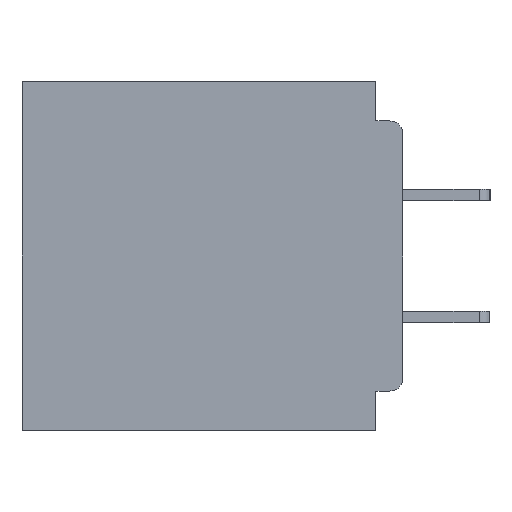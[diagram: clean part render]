
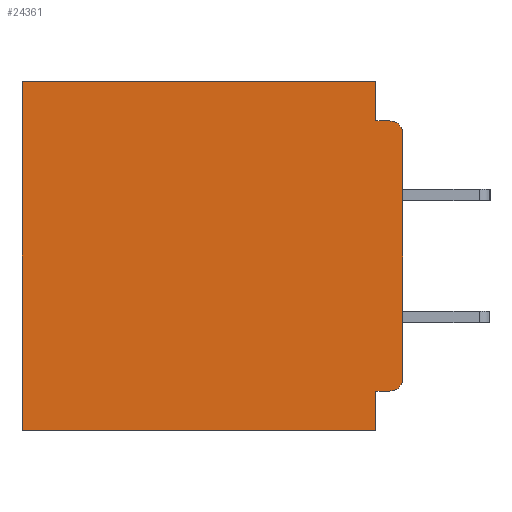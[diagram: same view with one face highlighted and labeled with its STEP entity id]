
A CAD part, left-side view. The second image highlights one B-rep face of the part: STEP entity #24361.
In plain terms, the highlighted planar face has unit normal (-1, 0, 0).
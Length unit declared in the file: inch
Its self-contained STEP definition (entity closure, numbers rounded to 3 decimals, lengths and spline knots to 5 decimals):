
#434 = EDGE_CURVE ( 'NONE', #15680, #1506, #31696, .T. ) ;
#1429 = CARTESIAN_POINT ( 'NONE',  ( 0.3, 0., -0.4 ) ) ;
#1449 = EDGE_CURVE ( 'NONE', #29071, #23700, #7052, .T. ) ;
#1506 = VERTEX_POINT ( 'NONE', #19476 ) ;
#1617 = DIRECTION ( 'NONE',  ( -1., 0., 0. ) ) ;
#1661 = CARTESIAN_POINT ( 'NONE',  ( 0.3, 0., -0.4 ) ) ;
#1756 = DIRECTION ( 'NONE',  ( 0., 0., -1. ) ) ;
#2538 = EDGE_LOOP ( 'NONE', ( #7887, #25222, #10624, #26122, #35601, #5634, #32492, #4267, #19746, #13804 ) ) ;
#2612 = CARTESIAN_POINT ( 'NONE',  ( 0.3, 0.031, -0.4 ) ) ;
#3013 = DIRECTION ( 'NONE',  ( -1., 0., 0. ) ) ;
#3930 = LINE ( 'NONE', #22100, #33946 ) ;
#4070 = EDGE_CURVE ( 'NONE', #23886, #24846, #15529, .T. ) ;
#4168 = EDGE_CURVE ( 'NONE', #24846, #30681, #34199, .T. ) ;
#4225 = CARTESIAN_POINT ( 'NONE',  ( 0.3, 0., -0.355 ) ) ;
#4267 = ORIENTED_EDGE ( 'NONE', *, *, #4168, .F. ) ;
#5488 = CARTESIAN_POINT ( 'NONE',  ( 0.3, 0., -0.045 ) ) ;
#5634 = ORIENTED_EDGE ( 'NONE', *, *, #24002, .T. ) ;
#5929 = DIRECTION ( 'NONE',  ( 0., 0., -1. ) ) ;
#6132 = LINE ( 'NONE', #1661, #36965 ) ;
#7052 = LINE ( 'NONE', #22260, #22573 ) ;
#7841 = VECTOR ( 'NONE', #13081, 39.37008 ) ;
#7887 = ORIENTED_EDGE ( 'NONE', *, *, #434, .F. ) ;
#8586 = AXIS2_PLACEMENT_3D ( 'NONE', #19026, #1617, #21970 ) ;
#8713 = DIRECTION ( 'NONE',  ( 0., 0., -1. ) ) ;
#9710 = VECTOR ( 'NONE', #11336, 39.37008 ) ;
#9947 = AXIS2_PLACEMENT_3D ( 'NONE', #20431, #3013, #23406 ) ;
#10624 = ORIENTED_EDGE ( 'NONE', *, *, #18194, .F. ) ;
#10672 = DIRECTION ( 'NONE',  ( 0., 0., -1. ) ) ;
#11080 = EDGE_CURVE ( 'NONE', #23886, #1506, #13443, .T. ) ;
#11336 = DIRECTION ( 'NONE',  ( 0., -1., 0. ) ) ;
#11985 = CIRCLE ( 'NONE', #8586, 0.015 ) ;
#12061 = CARTESIAN_POINT ( 'NONE',  ( 0.3, 0.031, -0.045 ) ) ;
#12838 = EDGE_CURVE ( 'NONE', #30681, #35003, #6132, .T. ) ;
#13081 = DIRECTION ( 'NONE',  ( 0., 1., 0. ) ) ;
#13393 = EDGE_CURVE ( 'NONE', #15680, #36923, #11985, .T. ) ;
#13443 = CIRCLE ( 'NONE', #9947, 0.015 ) ;
#13804 = ORIENTED_EDGE ( 'NONE', *, *, #11080, .T. ) ;
#15041 = PLANE ( 'NONE',  #25423 ) ;
#15529 = LINE ( 'NONE', #4225, #7841 ) ;
#15680 = VERTEX_POINT ( 'NONE', #17124 ) ;
#16155 = DIRECTION ( 'NONE',  ( 0., 1., 0. ) ) ;
#16560 = CARTESIAN_POINT ( 'NONE',  ( 0.3, 0.437, -0.4 ) ) ;
#16806 = CARTESIAN_POINT ( 'NONE',  ( 0.3, 0.015, -0.045 ) ) ;
#17124 = CARTESIAN_POINT ( 'NONE',  ( 0.3, 0., -0.06 ) ) ;
#17979 = DIRECTION ( 'NONE',  ( 0., 0., -1. ) ) ;
#18194 = EDGE_CURVE ( 'NONE', #23700, #36923, #18333, .T. ) ;
#18333 = LINE ( 'NONE', #5488, #9710 ) ;
#18659 = LINE ( 'NONE', #25003, #19580 ) ;
#19026 = CARTESIAN_POINT ( 'NONE',  ( 0.3, 0.015, -0.06 ) ) ;
#19195 = DIRECTION ( 'NONE',  ( 0., 1., 0. ) ) ;
#19476 = CARTESIAN_POINT ( 'NONE',  ( 0.3, 0., -0.34 ) ) ;
#19580 = VECTOR ( 'NONE', #16155, 39.37008 ) ;
#19746 = ORIENTED_EDGE ( 'NONE', *, *, #4070, .F. ) ;
#20431 = CARTESIAN_POINT ( 'NONE',  ( 0.3, 0.015, -0.34 ) ) ;
#21184 = FACE_OUTER_BOUND ( 'NONE', #2538, .T. ) ;
#21970 = DIRECTION ( 'NONE',  ( 0., 0., -1. ) ) ;
#22100 = CARTESIAN_POINT ( 'NONE',  ( 0.3, 0.437, -0.4 ) ) ;
#22260 = CARTESIAN_POINT ( 'NONE',  ( 0.3, 0.031, 0. ) ) ;
#22568 = VERTEX_POINT ( 'NONE', #23753 ) ;
#22573 = VECTOR ( 'NONE', #10672, 39.37008 ) ;
#23406 = DIRECTION ( 'NONE',  ( 0., 0., -1. ) ) ;
#23700 = VERTEX_POINT ( 'NONE', #12061 ) ;
#23753 = CARTESIAN_POINT ( 'NONE',  ( 0.3, 0.437, 0. ) ) ;
#23886 = VERTEX_POINT ( 'NONE', #33165 ) ;
#23971 = VECTOR ( 'NONE', #8713, 39.37008 ) ;
#24002 = EDGE_CURVE ( 'NONE', #22568, #35003, #3930, .T. ) ;
#24361 = ADVANCED_FACE ( 'NONE', ( #21184 ), #15041, .F. ) ;
#24846 = VERTEX_POINT ( 'NONE', #29202 ) ;
#25003 = CARTESIAN_POINT ( 'NONE',  ( 0.3, 0., 0. ) ) ;
#25222 = ORIENTED_EDGE ( 'NONE', *, *, #13393, .T. ) ;
#25423 = AXIS2_PLACEMENT_3D ( 'NONE', #29629, #35380, #17979 ) ;
#26122 = ORIENTED_EDGE ( 'NONE', *, *, #1449, .F. ) ;
#26502 = VECTOR ( 'NONE', #5929, 39.37008 ) ;
#29071 = VERTEX_POINT ( 'NONE', #32996 ) ;
#29202 = CARTESIAN_POINT ( 'NONE',  ( 0.3, 0.031, -0.355 ) ) ;
#29361 = EDGE_CURVE ( 'NONE', #29071, #22568, #18659, .T. ) ;
#29629 = CARTESIAN_POINT ( 'NONE',  ( 0.3, 0., -0.4 ) ) ;
#30681 = VERTEX_POINT ( 'NONE', #37246 ) ;
#31696 = LINE ( 'NONE', #1429, #23971 ) ;
#32492 = ORIENTED_EDGE ( 'NONE', *, *, #12838, .F. ) ;
#32996 = CARTESIAN_POINT ( 'NONE',  ( 0.3, 0.031, 0. ) ) ;
#33165 = CARTESIAN_POINT ( 'NONE',  ( 0.3, 0.015, -0.355 ) ) ;
#33946 = VECTOR ( 'NONE', #1756, 39.37008 ) ;
#34199 = LINE ( 'NONE', #2612, #26502 ) ;
#35003 = VERTEX_POINT ( 'NONE', #16560 ) ;
#35380 = DIRECTION ( 'NONE',  ( 1., 0., 0. ) ) ;
#35601 = ORIENTED_EDGE ( 'NONE', *, *, #29361, .T. ) ;
#36923 = VERTEX_POINT ( 'NONE', #16806 ) ;
#36965 = VECTOR ( 'NONE', #19195, 39.37008 ) ;
#37246 = CARTESIAN_POINT ( 'NONE',  ( 0.3, 0.031, -0.4 ) ) ;
